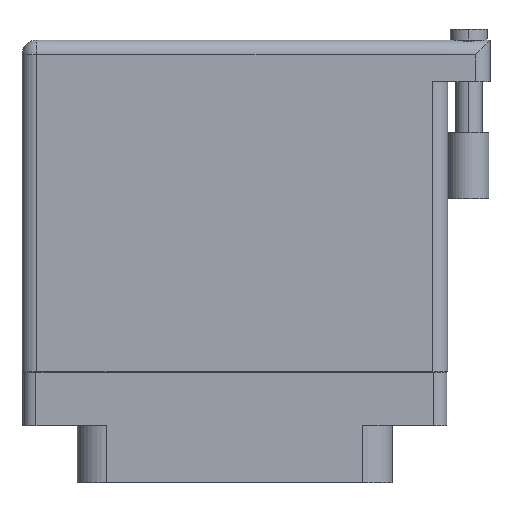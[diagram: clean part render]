
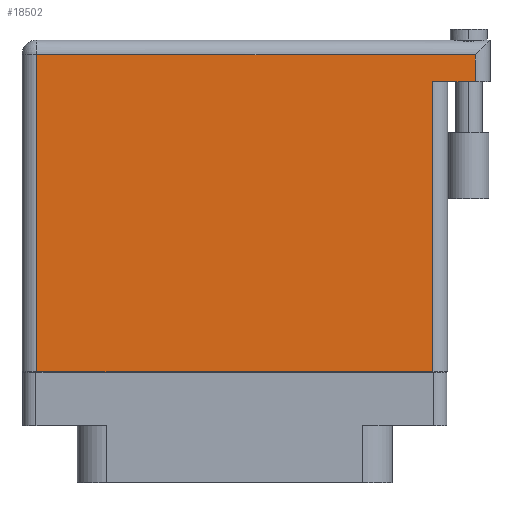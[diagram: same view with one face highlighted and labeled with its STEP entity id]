
A CAD part, front view. The second image highlights one B-rep face of the part: STEP entity #18502.
In plain terms, the highlighted face is planar.
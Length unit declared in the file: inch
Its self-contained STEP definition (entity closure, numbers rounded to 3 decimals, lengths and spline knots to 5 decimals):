
#269 = ORIENTED_EDGE ( 'NONE', *, *, #27387, .T. ) ;
#383 = CARTESIAN_POINT ( 'NONE',  ( 1.204, 1.269, 0.4495 ) ) ;
#588 = VECTOR ( 'NONE', #16908, 39.37008 ) ;
#987 = CARTESIAN_POINT ( 'NONE',  ( 0.934, 1.269, 0.4495 ) ) ;
#1631 = CARTESIAN_POINT ( 'NONE',  ( -0.934, -0.1, 0.4495 ) ) ;
#2062 = VECTOR ( 'NONE', #33524, 39.37008 ) ;
#2156 = CARTESIAN_POINT ( 'NONE',  ( 0.934, 1.269, 0.4495 ) ) ;
#2921 = VERTEX_POINT ( 'NONE', #4391 ) ;
#3638 = LINE ( 'NONE', #1631, #19265 ) ;
#4196 = DIRECTION ( 'NONE',  ( 0., -1., 0. ) ) ;
#4391 = CARTESIAN_POINT ( 'NONE',  ( 0.934, -0.1, 0.4495 ) ) ;
#4779 = FACE_OUTER_BOUND ( 'NONE', #24130, .T. ) ;
#5046 = EDGE_CURVE ( 'NONE', #32573, #5860, #22083, .T. ) ;
#5860 = VERTEX_POINT ( 'NONE', #20499 ) ;
#7399 = ORIENTED_EDGE ( 'NONE', *, *, #17939, .T. ) ;
#7794 = DIRECTION ( 'NONE',  ( 1., 0., 0. ) ) ;
#8492 = LINE ( 'NONE', #987, #13689 ) ;
#8842 = LINE ( 'NONE', #383, #588 ) ;
#11639 = VERTEX_POINT ( 'NONE', #14825 ) ;
#12286 = VECTOR ( 'NONE', #29727, 39.37008 ) ;
#13099 = PLANE ( 'NONE',  #26665 ) ;
#13215 = CARTESIAN_POINT ( 'NONE',  ( -1.004, 1.466, 0.4495 ) ) ;
#13689 = VECTOR ( 'NONE', #25967, 39.37008 ) ;
#14523 = VERTEX_POINT ( 'NONE', #24624 ) ;
#14774 = EDGE_CURVE ( 'NONE', #5860, #11639, #29367, .T. ) ;
#14825 = CARTESIAN_POINT ( 'NONE',  ( -0.934, 1.396, 0.4495 ) ) ;
#15283 = ORIENTED_EDGE ( 'NONE', *, *, #28460, .T. ) ;
#16733 = CARTESIAN_POINT ( 'NONE',  ( 1.134, 1.269, 0.4495 ) ) ;
#16908 = DIRECTION ( 'NONE',  ( -1., 0., 0. ) ) ;
#17939 = EDGE_CURVE ( 'NONE', #14523, #2921, #26958, .T. ) ;
#18502 = ADVANCED_FACE ( 'NONE', ( #4779 ), #13099, .F. ) ;
#18688 = DIRECTION ( 'NONE',  ( 0., 0., -1. ) ) ;
#19265 = VECTOR ( 'NONE', #4196, 39.37008 ) ;
#19633 = VECTOR ( 'NONE', #7794, 39.37008 ) ;
#20113 = ORIENTED_EDGE ( 'NONE', *, *, #5046, .T. ) ;
#20499 = CARTESIAN_POINT ( 'NONE',  ( 1.134, 1.396, 0.4495 ) ) ;
#21328 = ORIENTED_EDGE ( 'NONE', *, *, #14774, .T. ) ;
#21617 = CARTESIAN_POINT ( 'NONE',  ( -1.004, -0.1, 0.4495 ) ) ;
#22083 = LINE ( 'NONE', #29609, #12286 ) ;
#23895 = ORIENTED_EDGE ( 'NONE', *, *, #24434, .F. ) ;
#24130 = EDGE_LOOP ( 'NONE', ( #7399, #269, #23895, #20113, #21328, #15283 ) ) ;
#24434 = EDGE_CURVE ( 'NONE', #32573, #34160, #8842, .T. ) ;
#24624 = CARTESIAN_POINT ( 'NONE',  ( -0.934, -0.1, 0.4495 ) ) ;
#24925 = CARTESIAN_POINT ( 'NONE',  ( -1.004, 1.396, 0.4495 ) ) ;
#25967 = DIRECTION ( 'NONE',  ( 0., 1., 0. ) ) ;
#26665 = AXIS2_PLACEMENT_3D ( 'NONE', #13215, #18688, #32561 ) ;
#26958 = LINE ( 'NONE', #21617, #19633 ) ;
#27387 = EDGE_CURVE ( 'NONE', #2921, #34160, #8492, .T. ) ;
#28460 = EDGE_CURVE ( 'NONE', #11639, #14523, #3638, .T. ) ;
#29367 = LINE ( 'NONE', #24925, #2062 ) ;
#29609 = CARTESIAN_POINT ( 'NONE',  ( 1.134, 1.466, 0.4495 ) ) ;
#29727 = DIRECTION ( 'NONE',  ( 0., 1., 0. ) ) ;
#32561 = DIRECTION ( 'NONE',  ( -1., 0., 0. ) ) ;
#32573 = VERTEX_POINT ( 'NONE', #16733 ) ;
#33524 = DIRECTION ( 'NONE',  ( -1., 0., 0. ) ) ;
#34160 = VERTEX_POINT ( 'NONE', #2156 ) ;
